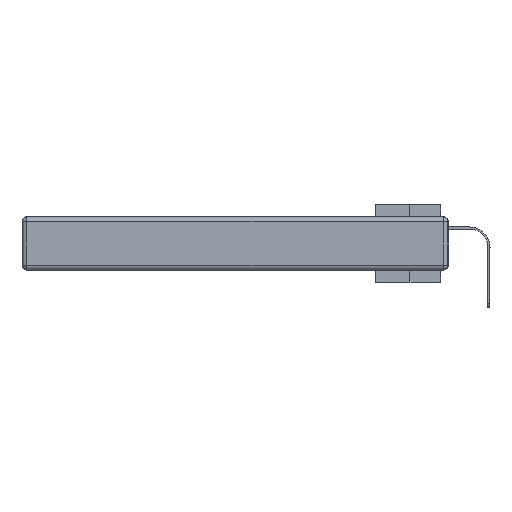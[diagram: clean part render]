
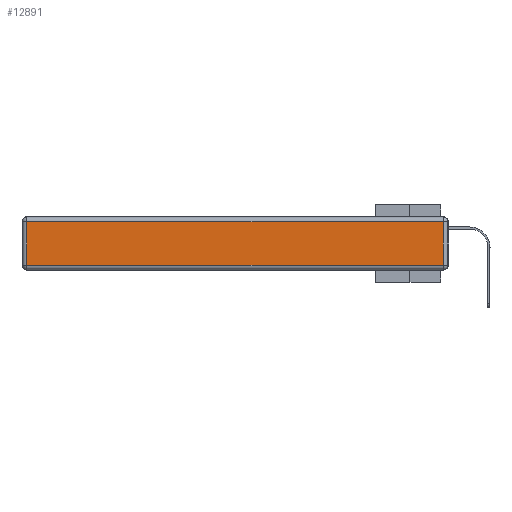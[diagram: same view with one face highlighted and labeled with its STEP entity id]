
A CAD part, left-side view. The second image highlights one B-rep face of the part: STEP entity #12891.
In plain terms, the highlighted planar face has unit normal (-1, 0, 0).
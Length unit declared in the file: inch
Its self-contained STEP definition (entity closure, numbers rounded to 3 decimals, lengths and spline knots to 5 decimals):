
#846 = DIRECTION ( 'NONE',  ( 0., 0., 1. ) ) ;
#1058 = EDGE_CURVE ( 'NONE', #19473, #28550, #21610, .T. ) ;
#1622 = DIRECTION ( 'NONE',  ( 0., 1., 0. ) ) ;
#2911 = PLANE ( 'NONE',  #24280 ) ;
#4186 = LINE ( 'NONE', #19898, #29420 ) ;
#4394 = EDGE_CURVE ( 'NONE', #13556, #19473, #22600, .T. ) ;
#5888 = CARTESIAN_POINT ( 'NONE',  ( 0., 0.03, -0.343 ) ) ;
#7478 = CARTESIAN_POINT ( 'NONE',  ( 0., 0.03, -0.03 ) ) ;
#7975 = CARTESIAN_POINT ( 'NONE',  ( 0., 2.72, -0.03 ) ) ;
#9562 = EDGE_CURVE ( 'NONE', #17071, #13556, #27629, .T. ) ;
#10933 = CARTESIAN_POINT ( 'NONE',  ( 0., 0., -0.343 ) ) ;
#12382 = VECTOR ( 'NONE', #18895, 39.37008 ) ;
#12891 = ADVANCED_FACE ( 'NONE', ( #31772 ), #2911, .T. ) ;
#13123 = ORIENTED_EDGE ( 'NONE', *, *, #1058, .T. ) ;
#13556 = VERTEX_POINT ( 'NONE', #22277 ) ;
#14651 = DIRECTION ( 'NONE',  ( 0., 0., -1. ) ) ;
#14755 = DIRECTION ( 'NONE',  ( 0., -1., 0. ) ) ;
#16139 = VECTOR ( 'NONE', #14651, 39.37008 ) ;
#16409 = DIRECTION ( 'NONE',  ( -1., 0., 0. ) ) ;
#17071 = VERTEX_POINT ( 'NONE', #7975 ) ;
#18895 = DIRECTION ( 'NONE',  ( 0., 0., 1. ) ) ;
#19473 = VERTEX_POINT ( 'NONE', #20914 ) ;
#19585 = ORIENTED_EDGE ( 'NONE', *, *, #4394, .T. ) ;
#19898 = CARTESIAN_POINT ( 'NONE',  ( 0., 2.75, -0.03 ) ) ;
#20546 = VECTOR ( 'NONE', #14755, 39.37008 ) ;
#20914 = CARTESIAN_POINT ( 'NONE',  ( 0., 0.03, -0.313 ) ) ;
#21610 = LINE ( 'NONE', #5888, #12382 ) ;
#22277 = CARTESIAN_POINT ( 'NONE',  ( 0., 2.72, -0.313 ) ) ;
#22439 = CARTESIAN_POINT ( 'NONE',  ( 0., 0., -0.313 ) ) ;
#22600 = LINE ( 'NONE', #22439, #20546 ) ;
#23676 = ORIENTED_EDGE ( 'NONE', *, *, #30468, .T. ) ;
#24280 = AXIS2_PLACEMENT_3D ( 'NONE', #10933, #16409, #846 ) ;
#27243 = ORIENTED_EDGE ( 'NONE', *, *, #9562, .T. ) ;
#27579 = EDGE_LOOP ( 'NONE', ( #19585, #13123, #23676, #27243 ) ) ;
#27629 = LINE ( 'NONE', #32752, #16139 ) ;
#28550 = VERTEX_POINT ( 'NONE', #7478 ) ;
#29420 = VECTOR ( 'NONE', #1622, 39.37008 ) ;
#30468 = EDGE_CURVE ( 'NONE', #28550, #17071, #4186, .T. ) ;
#31772 = FACE_OUTER_BOUND ( 'NONE', #27579, .T. ) ;
#32752 = CARTESIAN_POINT ( 'NONE',  ( 0., 2.72, -0.343 ) ) ;
